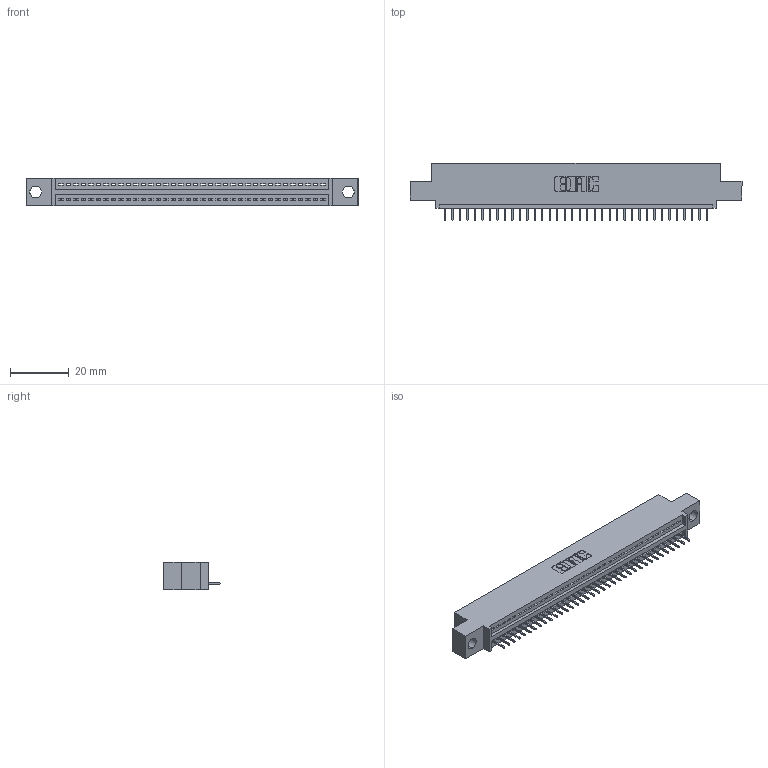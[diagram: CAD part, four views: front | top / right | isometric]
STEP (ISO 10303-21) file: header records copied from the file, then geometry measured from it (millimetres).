
FILE_DESCRIPTION (( 'STEP AP203' ), '1' );
FILE_NAME ('395-036-524-404.STEP', '2021-05-31T14:53:47', ( '' ), ( '' ), 'SwSTEP 2.0', 'SolidWorks 2020', '' );
FILE_SCHEMA (( 'CONFIG_CONTROL_DESIGN' ));
Length unit declared in the file: inch
Products named in the file (3): 395-036-524-404; 345 Part_0.110 Offset - 0.156 Dia-TI; 345-292-001_345-293-124
Assembly tree (37 placements, depth 2):
  395-036-524-404
    345 Part_0.110 Offset - 0.156 Dia-TI
    345-292-001_345-293-124  x36
Bounding box: 112.65 x 19.35 x 9.4 mm (x, y, z)
Volume: 10328.8 mm3; surface area: 13114.2 mm2
Topology: 37 solids, 37 shells, 2376 faces, 6869 edges, 4434 vertices
Faces by surface type: plane 1754, cylinder 622
Entity records: 28527 total; most frequent: CARTESIAN_POINT 4950, ORIENTED_EDGE 4918, DIRECTION 4331, EDGE_CURVE 2459, LINE 2187, VECTOR 2187, VERTEX_POINT 1634, AXIS2_PLACEMENT_3D 1072
